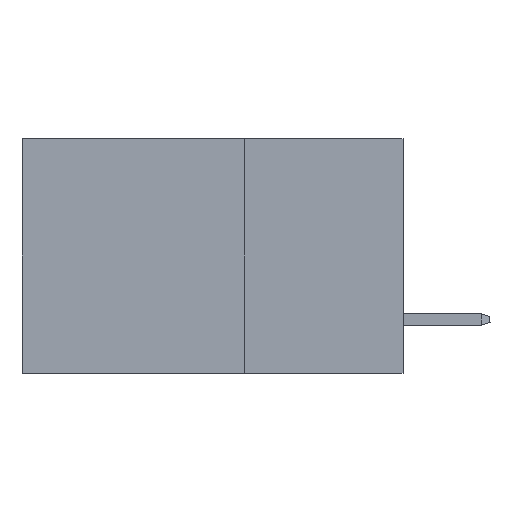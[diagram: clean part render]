
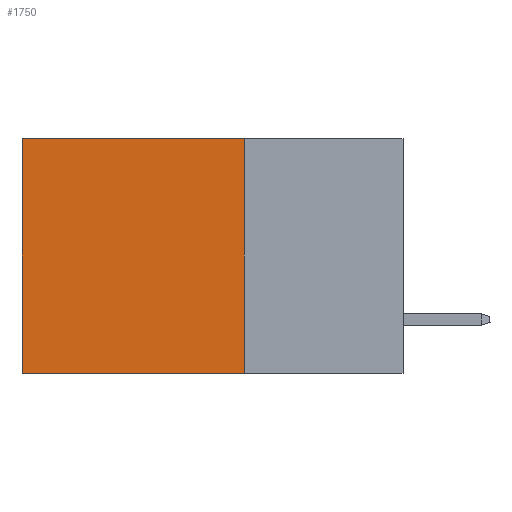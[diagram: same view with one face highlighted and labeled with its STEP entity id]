
A CAD part, left-side view. The second image highlights one B-rep face of the part: STEP entity #1750.
In plain terms, the highlighted planar face has unit normal (-1, 0, 0).
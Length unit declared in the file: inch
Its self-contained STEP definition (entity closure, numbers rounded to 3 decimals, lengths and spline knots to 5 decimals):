
#375 = VERTEX_POINT ( 'NONE', #10113 ) ;
#440 = LINE ( 'NONE', #4499, #4598 ) ;
#472 = VECTOR ( 'NONE', #11662, 39.37008 ) ;
#732 = CARTESIAN_POINT ( 'NONE',  ( 0.2875, 0.25, 0. ) ) ;
#1072 = LINE ( 'NONE', #11764, #2972 ) ;
#1456 = EDGE_CURVE ( 'NONE', #375, #3747, #13070, .T. ) ;
#1750 = ADVANCED_FACE ( 'NONE', ( #14922 ), #8132, .F. ) ;
#2094 = ORIENTED_EDGE ( 'NONE', *, *, #1456, .T. ) ;
#2330 = VERTEX_POINT ( 'NONE', #17345 ) ;
#2972 = VECTOR ( 'NONE', #14549, 39.37008 ) ;
#3367 = CARTESIAN_POINT ( 'NONE',  ( 0.2875, 0.6, -0.37 ) ) ;
#3415 = EDGE_CURVE ( 'NONE', #12971, #2330, #440, .T. ) ;
#3747 = VERTEX_POINT ( 'NONE', #3367 ) ;
#3780 = LINE ( 'NONE', #10703, #472 ) ;
#4499 = CARTESIAN_POINT ( 'NONE',  ( 0.2875, 0.25, 0. ) ) ;
#4598 = VECTOR ( 'NONE', #9063, 39.37008 ) ;
#5072 = EDGE_LOOP ( 'NONE', ( #2094, #15962, #6874, #14771 ) ) ;
#6255 = DIRECTION ( 'NONE',  ( 0., 0., -1. ) ) ;
#6798 = VECTOR ( 'NONE', #6255, 39.37008 ) ;
#6874 = ORIENTED_EDGE ( 'NONE', *, *, #3415, .F. ) ;
#6998 = CARTESIAN_POINT ( 'NONE',  ( 0.2875, 0.25, 0. ) ) ;
#8132 = PLANE ( 'NONE',  #16931 ) ;
#9063 = DIRECTION ( 'NONE',  ( 0., 0., -1. ) ) ;
#10113 = CARTESIAN_POINT ( 'NONE',  ( 0.2875, 0.6, 0. ) ) ;
#10441 = CARTESIAN_POINT ( 'NONE',  ( 0.2875, 0.6, 0. ) ) ;
#10578 = DIRECTION ( 'NONE',  ( 1., 0., 0. ) ) ;
#10703 = CARTESIAN_POINT ( 'NONE',  ( 0.2875, 0.25, 0. ) ) ;
#10917 = DIRECTION ( 'NONE',  ( 0., 0., -1. ) ) ;
#11662 = DIRECTION ( 'NONE',  ( 0., 1., 0. ) ) ;
#11764 = CARTESIAN_POINT ( 'NONE',  ( 0.2875, 0.25, -0.37 ) ) ;
#12971 = VERTEX_POINT ( 'NONE', #732 ) ;
#13070 = LINE ( 'NONE', #10441, #6798 ) ;
#13518 = EDGE_CURVE ( 'NONE', #12971, #375, #3780, .T. ) ;
#14549 = DIRECTION ( 'NONE',  ( 0., 1., 0. ) ) ;
#14771 = ORIENTED_EDGE ( 'NONE', *, *, #13518, .T. ) ;
#14922 = FACE_OUTER_BOUND ( 'NONE', #5072, .T. ) ;
#15962 = ORIENTED_EDGE ( 'NONE', *, *, #17336, .F. ) ;
#16931 = AXIS2_PLACEMENT_3D ( 'NONE', #6998, #10578, #10917 ) ;
#17336 = EDGE_CURVE ( 'NONE', #2330, #3747, #1072, .T. ) ;
#17345 = CARTESIAN_POINT ( 'NONE',  ( 0.2875, 0.25, -0.37 ) ) ;
